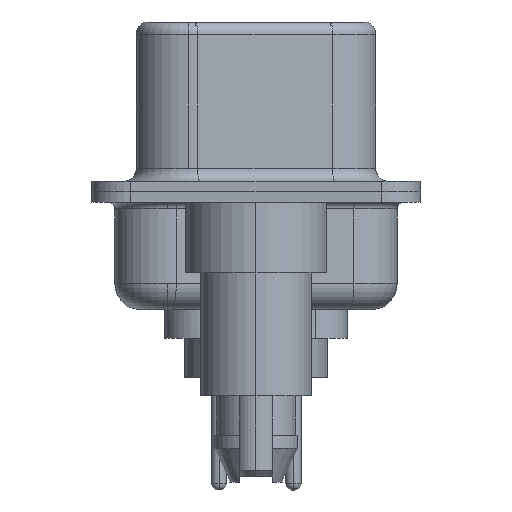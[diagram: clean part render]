
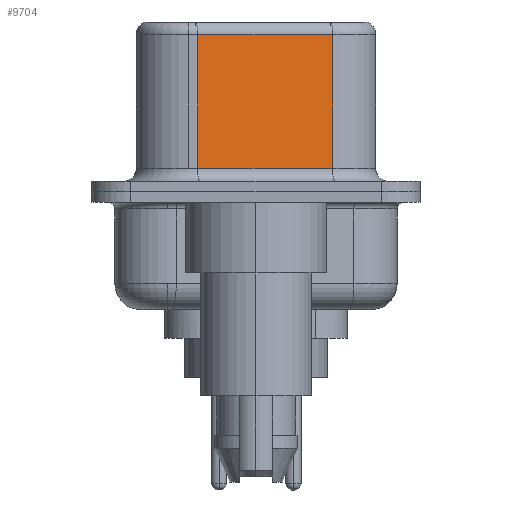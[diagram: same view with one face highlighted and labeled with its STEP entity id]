
A CAD part, left-side view. The second image highlights one B-rep face of the part: STEP entity #9704.
In plain terms, the highlighted planar face has unit normal (-0.985, -0.174, 0).
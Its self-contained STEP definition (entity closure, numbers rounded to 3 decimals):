
#379 = EDGE_CURVE ( 'NONE', #2069, #17244, #12999, .T. ) ;
#1083 = VERTEX_POINT ( 'NONE', #17442 ) ;
#2069 = VERTEX_POINT ( 'NONE', #7661 ) ;
#3086 = ORIENTED_EDGE ( 'NONE', *, *, #16880, .T. ) ;
#4159 = VECTOR ( 'NONE', #9022, 1000. ) ;
#4925 = CARTESIAN_POINT ( 'NONE',  ( 4.58, -2.927, 0.9 ) ) ;
#5363 = VECTOR ( 'NONE', #17130, 1000. ) ;
#7661 = CARTESIAN_POINT ( 'NONE',  ( 4.58, -2.927, 6.02 ) ) ;
#8205 = EDGE_CURVE ( 'NONE', #1083, #14912, #13460, .T. ) ;
#8290 = LINE ( 'NONE', #9086, #4159 ) ;
#8402 = PLANE ( 'NONE',  #14760 ) ;
#8470 = DIRECTION ( 'NONE',  ( -0.174, 0.985, 0. ) ) ;
#8759 = ORIENTED_EDGE ( 'NONE', *, *, #379, .T. ) ;
#9022 = DIRECTION ( 'NONE',  ( 0., 0., -1. ) ) ;
#9086 = CARTESIAN_POINT ( 'NONE',  ( 3.67, 2.233, 6.52 ) ) ;
#9220 = EDGE_CURVE ( 'NONE', #2069, #14912, #17016, .T. ) ;
#9704 = ADVANCED_FACE ( 'NONE', ( #13403 ), #8402, .F. ) ;
#10518 = CARTESIAN_POINT ( 'NONE',  ( 4.58, -2.927, 6.02 ) ) ;
#12946 = VECTOR ( 'NONE', #15001, 1000. ) ;
#12999 = LINE ( 'NONE', #10518, #13951 ) ;
#13403 = FACE_OUTER_BOUND ( 'NONE', #14342, .T. ) ;
#13460 = LINE ( 'NONE', #4925, #5363 ) ;
#13616 = ORIENTED_EDGE ( 'NONE', *, *, #9220, .F. ) ;
#13951 = VECTOR ( 'NONE', #19112, 1000. ) ;
#14342 = EDGE_LOOP ( 'NONE', ( #13616, #8759, #3086, #19703 ) ) ;
#14492 = CARTESIAN_POINT ( 'NONE',  ( 3.67, 2.233, 6.02 ) ) ;
#14499 = CARTESIAN_POINT ( 'NONE',  ( 4.58, -2.927, 6.52 ) ) ;
#14760 = AXIS2_PLACEMENT_3D ( 'NONE', #14499, #17591, #8470 ) ;
#14912 = VERTEX_POINT ( 'NONE', #17606 ) ;
#15001 = DIRECTION ( 'NONE',  ( 0., 0., -1. ) ) ;
#16880 = EDGE_CURVE ( 'NONE', #17244, #1083, #8290, .T. ) ;
#17016 = LINE ( 'NONE', #18016, #12946 ) ;
#17130 = DIRECTION ( 'NONE',  ( 0.174, -0.985, 0. ) ) ;
#17244 = VERTEX_POINT ( 'NONE', #14492 ) ;
#17442 = CARTESIAN_POINT ( 'NONE',  ( 3.67, 2.233, 0.9 ) ) ;
#17591 = DIRECTION ( 'NONE',  ( 0.985, 0.174, 0. ) ) ;
#17606 = CARTESIAN_POINT ( 'NONE',  ( 4.58, -2.927, 0.9 ) ) ;
#18016 = CARTESIAN_POINT ( 'NONE',  ( 4.58, -2.927, 6.52 ) ) ;
#19112 = DIRECTION ( 'NONE',  ( -0.174, 0.985, 0. ) ) ;
#19703 = ORIENTED_EDGE ( 'NONE', *, *, #8205, .T. ) ;
